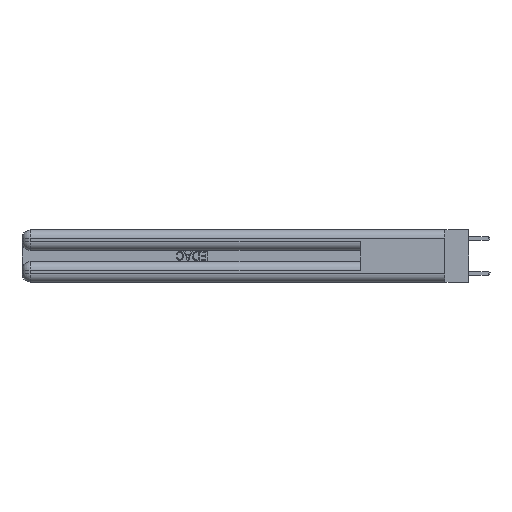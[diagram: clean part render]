
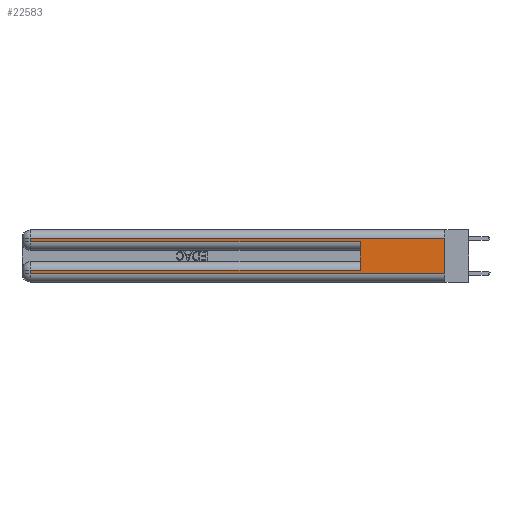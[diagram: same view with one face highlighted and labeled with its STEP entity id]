
A CAD part, left-side view. The second image highlights one B-rep face of the part: STEP entity #22583.
In plain terms, the highlighted planar face has unit normal (-1, 0, 0).
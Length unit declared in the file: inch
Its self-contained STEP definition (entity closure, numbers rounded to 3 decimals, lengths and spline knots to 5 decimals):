
#679 = EDGE_CURVE ( 'NONE', #4949, #22878, #21224, .T. ) ;
#707 = CARTESIAN_POINT ( 'NONE',  ( 0., 2.94, 0.37 ) ) ;
#1052 = CARTESIAN_POINT ( 'NONE',  ( 0., 0.6, 0.285 ) ) ;
#2363 = ORIENTED_EDGE ( 'NONE', *, *, #3827, .T. ) ;
#2715 = CARTESIAN_POINT ( 'NONE',  ( 0., 0.6, 0.085 ) ) ;
#3280 = CARTESIAN_POINT ( 'NONE',  ( 0., 2.94, 0.31 ) ) ;
#3440 = AXIS2_PLACEMENT_3D ( 'NONE', #15287, #9452, #31938 ) ;
#3814 = VERTEX_POINT ( 'NONE', #3864 ) ;
#3827 = EDGE_CURVE ( 'NONE', #19492, #3814, #20677, .T. ) ;
#3864 = CARTESIAN_POINT ( 'NONE',  ( 0., 0., 0.06 ) ) ;
#4246 = EDGE_CURVE ( 'NONE', #22878, #19492, #6090, .T. ) ;
#4408 = EDGE_CURVE ( 'NONE', #34154, #35139, #14337, .T. ) ;
#4949 = VERTEX_POINT ( 'NONE', #2715 ) ;
#4978 = CARTESIAN_POINT ( 'NONE',  ( 0., 0.6, 0.145 ) ) ;
#5828 = EDGE_CURVE ( 'NONE', #35139, #6655, #23587, .T. ) ;
#5986 = ORIENTED_EDGE ( 'NONE', *, *, #17231, .F. ) ;
#6090 = LINE ( 'NONE', #29130, #17935 ) ;
#6538 = CARTESIAN_POINT ( 'NONE',  ( 0., 0., 0.285 ) ) ;
#6655 = VERTEX_POINT ( 'NONE', #27042 ) ;
#7810 = DIRECTION ( 'NONE',  ( 0., -1., 0. ) ) ;
#9452 = DIRECTION ( 'NONE',  ( 1., 0., 0. ) ) ;
#10165 = VERTEX_POINT ( 'NONE', #1052 ) ;
#10847 = LINE ( 'NONE', #4978, #24999 ) ;
#11243 = VECTOR ( 'NONE', #35055, 39.37008 ) ;
#11318 = VECTOR ( 'NONE', #12265, 39.37008 ) ;
#11945 = EDGE_CURVE ( 'NONE', #4949, #10165, #10847, .T. ) ;
#11950 = CARTESIAN_POINT ( 'NONE',  ( 0., 0., 0.31 ) ) ;
#12265 = DIRECTION ( 'NONE',  ( 0., 0., -1. ) ) ;
#12877 = ORIENTED_EDGE ( 'NONE', *, *, #14306, .T. ) ;
#14306 = EDGE_CURVE ( 'NONE', #6655, #10165, #28505, .T. ) ;
#14337 = LINE ( 'NONE', #34001, #15622 ) ;
#15119 = LINE ( 'NONE', #26645, #25195 ) ;
#15287 = CARTESIAN_POINT ( 'NONE',  ( 0., 0., 0.37 ) ) ;
#15297 = ORIENTED_EDGE ( 'NONE', *, *, #679, .T. ) ;
#15622 = VECTOR ( 'NONE', #16992, 39.37008 ) ;
#15717 = ORIENTED_EDGE ( 'NONE', *, *, #11945, .F. ) ;
#15808 = EDGE_LOOP ( 'NONE', ( #5986, #25809, #19941, #12877, #15717, #15297, #27324, #2363 ) ) ;
#16992 = DIRECTION ( 'NONE',  ( 0., 1., 0. ) ) ;
#17231 = EDGE_CURVE ( 'NONE', #34154, #3814, #15119, .T. ) ;
#17864 = CARTESIAN_POINT ( 'NONE',  ( 0., 0., 0.06 ) ) ;
#17935 = VECTOR ( 'NONE', #26305, 39.37008 ) ;
#18037 = CARTESIAN_POINT ( 'NONE',  ( 0., 0., 0.085 ) ) ;
#18758 = VECTOR ( 'NONE', #7810, 39.37008 ) ;
#19492 = VERTEX_POINT ( 'NONE', #35812 ) ;
#19941 = ORIENTED_EDGE ( 'NONE', *, *, #5828, .T. ) ;
#20405 = FACE_OUTER_BOUND ( 'NONE', #15808, .T. ) ;
#20586 = PLANE ( 'NONE',  #3440 ) ;
#20677 = LINE ( 'NONE', #17864, #18758 ) ;
#21224 = LINE ( 'NONE', #18037, #34095 ) ;
#21899 = DIRECTION ( 'NONE',  ( 0., 0., -1. ) ) ;
#22583 = ADVANCED_FACE ( 'NONE', ( #20405 ), #20586, .F. ) ;
#22878 = VERTEX_POINT ( 'NONE', #31705 ) ;
#23587 = LINE ( 'NONE', #707, #11318 ) ;
#24999 = VECTOR ( 'NONE', #33149, 39.37008 ) ;
#25195 = VECTOR ( 'NONE', #21899, 39.37008 ) ;
#25809 = ORIENTED_EDGE ( 'NONE', *, *, #4408, .T. ) ;
#26305 = DIRECTION ( 'NONE',  ( 0., 0., -1. ) ) ;
#26645 = CARTESIAN_POINT ( 'NONE',  ( 0., 0., 0.37 ) ) ;
#27042 = CARTESIAN_POINT ( 'NONE',  ( 0., 2.94, 0.285 ) ) ;
#27324 = ORIENTED_EDGE ( 'NONE', *, *, #4246, .T. ) ;
#28505 = LINE ( 'NONE', #6538, #11243 ) ;
#29130 = CARTESIAN_POINT ( 'NONE',  ( 0., 2.94, 0.37 ) ) ;
#31705 = CARTESIAN_POINT ( 'NONE',  ( 0., 2.94, 0.085 ) ) ;
#31938 = DIRECTION ( 'NONE',  ( 0., 0., -1. ) ) ;
#33129 = DIRECTION ( 'NONE',  ( 0., 1., 0. ) ) ;
#33149 = DIRECTION ( 'NONE',  ( 0., 0., 1. ) ) ;
#34001 = CARTESIAN_POINT ( 'NONE',  ( 0., 0., 0.31 ) ) ;
#34095 = VECTOR ( 'NONE', #33129, 39.37008 ) ;
#34154 = VERTEX_POINT ( 'NONE', #11950 ) ;
#35055 = DIRECTION ( 'NONE',  ( 0., -1., 0. ) ) ;
#35139 = VERTEX_POINT ( 'NONE', #3280 ) ;
#35812 = CARTESIAN_POINT ( 'NONE',  ( 0., 2.94, 0.06 ) ) ;
